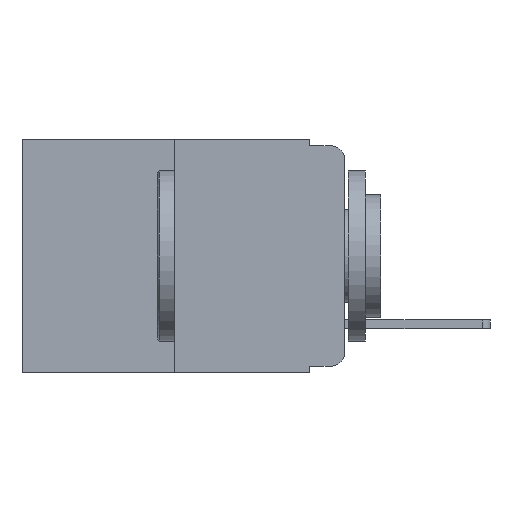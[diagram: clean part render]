
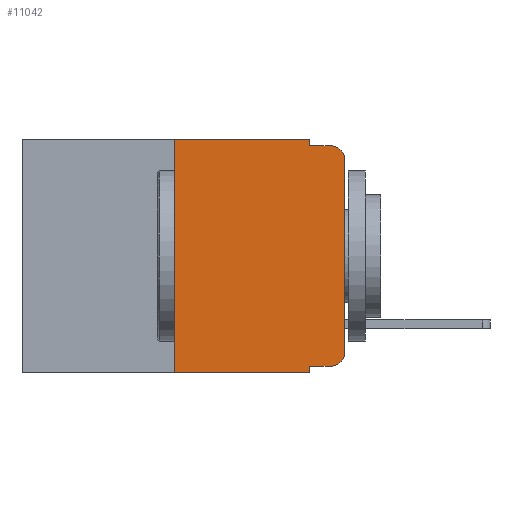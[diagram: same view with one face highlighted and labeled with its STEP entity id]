
A CAD part, left-side view. The second image highlights one B-rep face of the part: STEP entity #11042.
In plain terms, the highlighted planar face has unit normal (-1, 0, 0).
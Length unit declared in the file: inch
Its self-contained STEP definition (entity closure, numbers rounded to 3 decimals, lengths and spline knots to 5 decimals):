
#10 = CARTESIAN_POINT ( 'NONE',  ( 0., 0.02, -0.333 ) ) ;
#26 = CARTESIAN_POINT ( 'NONE',  ( 0., 0.473, 0. ) ) ;
#316 = CARTESIAN_POINT ( 'NONE',  ( 0., 0., 0. ) ) ;
#561 = CARTESIAN_POINT ( 'NONE',  ( 0., 0.051, 0. ) ) ;
#704 = ORIENTED_EDGE ( 'NONE', *, *, #9882, .T. ) ;
#1130 = DIRECTION ( 'NONE',  ( -1., 0., 0. ) ) ;
#1285 = LINE ( 'NONE', #9733, #7820 ) ;
#1325 = VERTEX_POINT ( 'NONE', #13445 ) ;
#1583 = LINE ( 'NONE', #5303, #10962 ) ;
#1625 = DIRECTION ( 'NONE',  ( 0., 0., 1. ) ) ;
#1656 = EDGE_CURVE ( 'NONE', #14140, #7315, #13964, .T. ) ;
#1801 = VERTEX_POINT ( 'NONE', #5777 ) ;
#2029 = LINE ( 'NONE', #316, #8378 ) ;
#2130 = VERTEX_POINT ( 'NONE', #15137 ) ;
#2160 = EDGE_CURVE ( 'NONE', #12451, #1325, #7826, .T. ) ;
#3212 = LINE ( 'NONE', #5580, #15492 ) ;
#3638 = EDGE_CURVE ( 'NONE', #12451, #8002, #10437, .T. ) ;
#3848 = DIRECTION ( 'NONE',  ( 0., 0., -1. ) ) ;
#4001 = LINE ( 'NONE', #561, #14967 ) ;
#4078 = DIRECTION ( 'NONE',  ( 0., 0., -1. ) ) ;
#4162 = CARTESIAN_POINT ( 'NONE',  ( 0., 0.02, -0.01 ) ) ;
#4220 = CARTESIAN_POINT ( 'NONE',  ( 0., 0.051, -0.343 ) ) ;
#4221 = ORIENTED_EDGE ( 'NONE', *, *, #4671, .T. ) ;
#4303 = DIRECTION ( 'NONE',  ( -1., 0., 0. ) ) ;
#4550 = CARTESIAN_POINT ( 'NONE',  ( 0., 0.25, 0. ) ) ;
#4671 = EDGE_CURVE ( 'NONE', #1801, #14866, #9266, .T. ) ;
#5303 = CARTESIAN_POINT ( 'NONE',  ( 0., 0.051, -0.333 ) ) ;
#5580 = CARTESIAN_POINT ( 'NONE',  ( 0., 0.473, 0. ) ) ;
#5777 = CARTESIAN_POINT ( 'NONE',  ( 0., 0., -0.03 ) ) ;
#6010 = CARTESIAN_POINT ( 'NONE',  ( 0., 0.473, -0.343 ) ) ;
#6148 = DIRECTION ( 'NONE',  ( 0., -1., 0. ) ) ;
#6553 = ORIENTED_EDGE ( 'NONE', *, *, #7419, .F. ) ;
#6697 = CARTESIAN_POINT ( 'NONE',  ( 0., 0.051, -0.01 ) ) ;
#6743 = VERTEX_POINT ( 'NONE', #6697 ) ;
#7219 = VECTOR ( 'NONE', #6148, 39.37008 ) ;
#7315 = VERTEX_POINT ( 'NONE', #11430 ) ;
#7419 = EDGE_CURVE ( 'NONE', #9175, #8002, #4001, .T. ) ;
#7475 = DIRECTION ( 'NONE',  ( 0., 0., 1. ) ) ;
#7795 = CARTESIAN_POINT ( 'NONE',  ( 0., 0.02, -0.313 ) ) ;
#7820 = VECTOR ( 'NONE', #10933, 39.37008 ) ;
#7826 = LINE ( 'NONE', #4550, #11824 ) ;
#7850 = ORIENTED_EDGE ( 'NONE', *, *, #11187, .F. ) ;
#7968 = DIRECTION ( 'NONE',  ( 0., 0., -1. ) ) ;
#8002 = VERTEX_POINT ( 'NONE', #4220 ) ;
#8045 = VECTOR ( 'NONE', #13701, 39.37008 ) ;
#8378 = VECTOR ( 'NONE', #1625, 39.37008 ) ;
#8428 = EDGE_CURVE ( 'NONE', #7315, #1801, #2029, .T. ) ;
#8574 = EDGE_CURVE ( 'NONE', #1325, #2130, #3212, .T. ) ;
#8613 = ORIENTED_EDGE ( 'NONE', *, *, #8574, .F. ) ;
#8645 = PLANE ( 'NONE',  #14040 ) ;
#9175 = VERTEX_POINT ( 'NONE', #15596 ) ;
#9233 = DIRECTION ( 'NONE',  ( 0., -1., 0. ) ) ;
#9266 = CIRCLE ( 'NONE', #12645, 0.02 ) ;
#9592 = ORIENTED_EDGE ( 'NONE', *, *, #8428, .T. ) ;
#9733 = CARTESIAN_POINT ( 'NONE',  ( 0., 0.051, 0. ) ) ;
#9882 = EDGE_CURVE ( 'NONE', #9175, #14140, #1583, .T. ) ;
#10007 = EDGE_LOOP ( 'NONE', ( #9592, #4221, #7850, #14127, #8613, #15173, #15530, #6553, #704, #13967 ) ) ;
#10150 = CARTESIAN_POINT ( 'NONE',  ( 0., 0.25, -0.343 ) ) ;
#10437 = LINE ( 'NONE', #6010, #7219 ) ;
#10527 = CARTESIAN_POINT ( 'NONE',  ( 0., 0.02, -0.03 ) ) ;
#10933 = DIRECTION ( 'NONE',  ( 0., 0., -1. ) ) ;
#10962 = VECTOR ( 'NONE', #13637, 39.37008 ) ;
#11042 = ADVANCED_FACE ( 'NONE', ( #13442 ), #8645, .F. ) ;
#11146 = DIRECTION ( 'NONE',  ( 1., 0., 0. ) ) ;
#11187 = EDGE_CURVE ( 'NONE', #6743, #14866, #11298, .T. ) ;
#11298 = LINE ( 'NONE', #12552, #8045 ) ;
#11430 = CARTESIAN_POINT ( 'NONE',  ( 0., 0., -0.313 ) ) ;
#11824 = VECTOR ( 'NONE', #7475, 39.37008 ) ;
#12247 = EDGE_CURVE ( 'NONE', #2130, #6743, #1285, .T. ) ;
#12451 = VERTEX_POINT ( 'NONE', #10150 ) ;
#12552 = CARTESIAN_POINT ( 'NONE',  ( 0., 0.051, -0.01 ) ) ;
#12645 = AXIS2_PLACEMENT_3D ( 'NONE', #10527, #1130, #14920 ) ;
#13442 = FACE_OUTER_BOUND ( 'NONE', #10007, .T. ) ;
#13445 = CARTESIAN_POINT ( 'NONE',  ( 0., 0.25, 0. ) ) ;
#13637 = DIRECTION ( 'NONE',  ( 0., -1., 0. ) ) ;
#13701 = DIRECTION ( 'NONE',  ( 0., -1., 0. ) ) ;
#13962 = AXIS2_PLACEMENT_3D ( 'NONE', #7795, #4303, #4078 ) ;
#13964 = CIRCLE ( 'NONE', #13962, 0.02 ) ;
#13967 = ORIENTED_EDGE ( 'NONE', *, *, #1656, .T. ) ;
#14040 = AXIS2_PLACEMENT_3D ( 'NONE', #26, #11146, #3848 ) ;
#14127 = ORIENTED_EDGE ( 'NONE', *, *, #12247, .F. ) ;
#14140 = VERTEX_POINT ( 'NONE', #10 ) ;
#14866 = VERTEX_POINT ( 'NONE', #4162 ) ;
#14920 = DIRECTION ( 'NONE',  ( 0., 0., -1. ) ) ;
#14967 = VECTOR ( 'NONE', #7968, 39.37008 ) ;
#15137 = CARTESIAN_POINT ( 'NONE',  ( 0., 0.051, 0. ) ) ;
#15173 = ORIENTED_EDGE ( 'NONE', *, *, #2160, .F. ) ;
#15492 = VECTOR ( 'NONE', #9233, 39.37008 ) ;
#15530 = ORIENTED_EDGE ( 'NONE', *, *, #3638, .T. ) ;
#15596 = CARTESIAN_POINT ( 'NONE',  ( 0., 0.051, -0.333 ) ) ;
